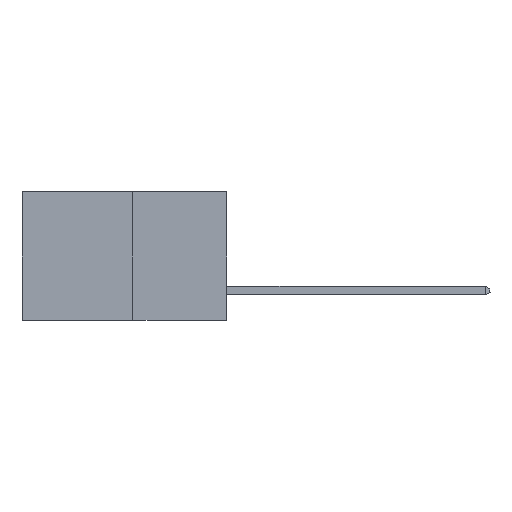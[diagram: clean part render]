
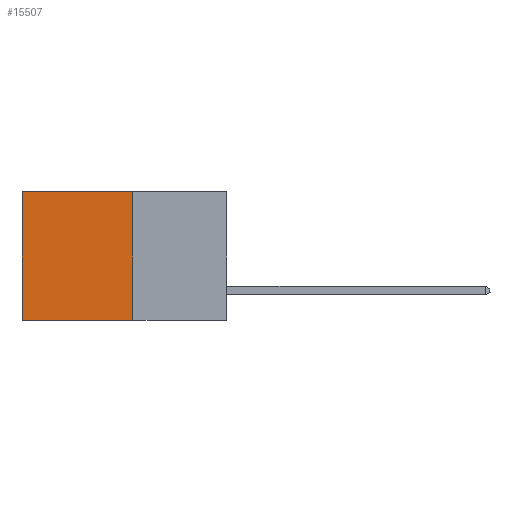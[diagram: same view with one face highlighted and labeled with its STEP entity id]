
A CAD part, left-side view. The second image highlights one B-rep face of the part: STEP entity #15507.
In plain terms, the highlighted planar face has unit normal (-1, 0, 0).
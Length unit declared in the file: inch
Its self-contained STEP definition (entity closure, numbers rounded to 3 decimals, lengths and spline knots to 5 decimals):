
#2136 = CARTESIAN_POINT ( 'NONE',  ( 0.277, 0.27, 0. ) ) ;
#2138 = LINE ( 'NONE', #18329, #13590 ) ;
#2201 = EDGE_CURVE ( 'NONE', #13920, #9718, #13915, .T. ) ;
#2276 = FACE_OUTER_BOUND ( 'NONE', #14249, .T. ) ;
#2457 = VECTOR ( 'NONE', #11874, 39.37008 ) ;
#2972 = ORIENTED_EDGE ( 'NONE', *, *, #8537, .F. ) ;
#3479 = CARTESIAN_POINT ( 'NONE',  ( 0.277, 0.27, -0.37 ) ) ;
#4653 = PLANE ( 'NONE',  #14721 ) ;
#6723 = ORIENTED_EDGE ( 'NONE', *, *, #2201, .T. ) ;
#6926 = VECTOR ( 'NONE', #7933, 39.37008 ) ;
#7374 = LINE ( 'NONE', #3479, #6926 ) ;
#7381 = VERTEX_POINT ( 'NONE', #16109 ) ;
#7419 = VERTEX_POINT ( 'NONE', #8737 ) ;
#7603 = DIRECTION ( 'NONE',  ( 0., 0., -1. ) ) ;
#7933 = DIRECTION ( 'NONE',  ( 0., 1., 0. ) ) ;
#8537 = EDGE_CURVE ( 'NONE', #13920, #7381, #2138, .T. ) ;
#8634 = EDGE_CURVE ( 'NONE', #9718, #7419, #12664, .T. ) ;
#8737 = CARTESIAN_POINT ( 'NONE',  ( 0.277, 0.59, -0.37 ) ) ;
#9718 = VERTEX_POINT ( 'NONE', #11772 ) ;
#11237 = CARTESIAN_POINT ( 'NONE',  ( 0.277, 0.27, 0. ) ) ;
#11772 = CARTESIAN_POINT ( 'NONE',  ( 0.277, 0.59, 0. ) ) ;
#11874 = DIRECTION ( 'NONE',  ( 0., 1., 0. ) ) ;
#12664 = LINE ( 'NONE', #15596, #15658 ) ;
#13590 = VECTOR ( 'NONE', #18312, 39.37008 ) ;
#13915 = LINE ( 'NONE', #2136, #2457 ) ;
#13920 = VERTEX_POINT ( 'NONE', #11237 ) ;
#14210 = ORIENTED_EDGE ( 'NONE', *, *, #15660, .F. ) ;
#14249 = EDGE_LOOP ( 'NONE', ( #17791, #14210, #2972, #6723 ) ) ;
#14721 = AXIS2_PLACEMENT_3D ( 'NONE', #15066, #16533, #7603 ) ;
#15066 = CARTESIAN_POINT ( 'NONE',  ( 0.277, 0.27, -0.37 ) ) ;
#15507 = ADVANCED_FACE ( 'NONE', ( #2276 ), #4653, .F. ) ;
#15560 = DIRECTION ( 'NONE',  ( 0., 0., -1. ) ) ;
#15596 = CARTESIAN_POINT ( 'NONE',  ( 0.277, 0.59, -0.37 ) ) ;
#15658 = VECTOR ( 'NONE', #15560, 39.37008 ) ;
#15660 = EDGE_CURVE ( 'NONE', #7381, #7419, #7374, .T. ) ;
#16109 = CARTESIAN_POINT ( 'NONE',  ( 0.277, 0.27, -0.37 ) ) ;
#16533 = DIRECTION ( 'NONE',  ( 1., 0., 0. ) ) ;
#17791 = ORIENTED_EDGE ( 'NONE', *, *, #8634, .T. ) ;
#18312 = DIRECTION ( 'NONE',  ( 0., 0., -1. ) ) ;
#18329 = CARTESIAN_POINT ( 'NONE',  ( 0.277, 0.27, -0.37 ) ) ;
